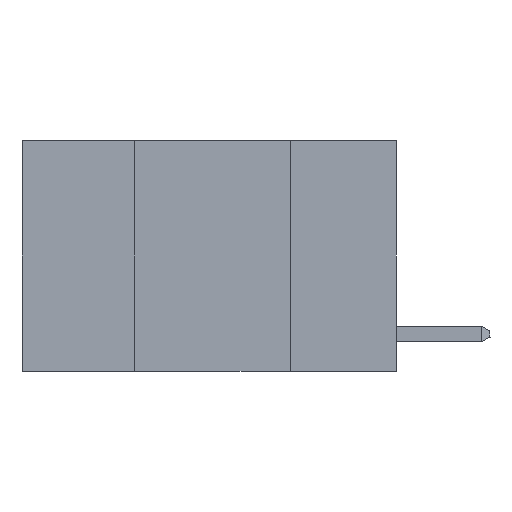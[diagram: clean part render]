
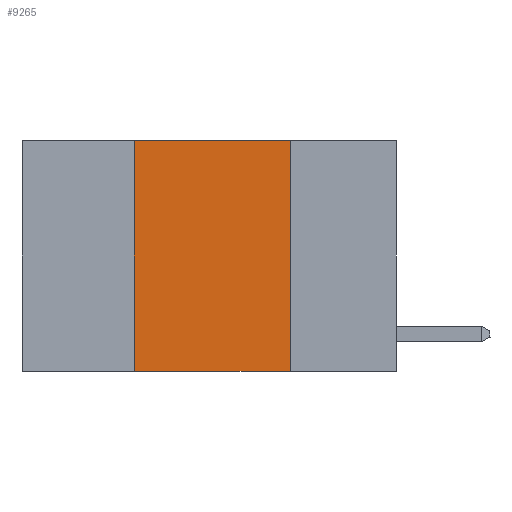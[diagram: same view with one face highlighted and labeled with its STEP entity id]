
A CAD part, left-side view. The second image highlights one B-rep face of the part: STEP entity #9265.
In plain terms, the highlighted planar face has unit normal (-1, 0, 0).
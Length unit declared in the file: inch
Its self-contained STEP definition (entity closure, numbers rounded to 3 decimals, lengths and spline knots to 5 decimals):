
#1022 = EDGE_CURVE ( 'NONE', #4609, #9097, #18171, .T. ) ;
#2296 = ORIENTED_EDGE ( 'NONE', *, *, #17796, .F. ) ;
#2890 = CARTESIAN_POINT ( 'NONE',  ( 0., 0.6, 0. ) ) ;
#3332 = VECTOR ( 'NONE', #21594, 39.37008 ) ;
#4609 = VERTEX_POINT ( 'NONE', #22070 ) ;
#4688 = CARTESIAN_POINT ( 'NONE',  ( 0., 0.42, 0. ) ) ;
#4901 = EDGE_LOOP ( 'NONE', ( #20134, #12432, #2296, #8765 ) ) ;
#5669 = LINE ( 'NONE', #23611, #23332 ) ;
#5858 = DIRECTION ( 'NONE',  ( 0., 0., -1. ) ) ;
#7520 = EDGE_CURVE ( 'NONE', #20606, #9097, #5669, .T. ) ;
#8765 = ORIENTED_EDGE ( 'NONE', *, *, #1022, .T. ) ;
#9097 = VERTEX_POINT ( 'NONE', #20006 ) ;
#9265 = ADVANCED_FACE ( 'NONE', ( #14627 ), #12189, .F. ) ;
#9330 = VECTOR ( 'NONE', #25806, 39.37008 ) ;
#9952 = VECTOR ( 'NONE', #20990, 39.37008 ) ;
#10067 = VERTEX_POINT ( 'NONE', #13952 ) ;
#10439 = DIRECTION ( 'NONE',  ( 1., 0., 0. ) ) ;
#11130 = LINE ( 'NONE', #2890, #9330 ) ;
#11728 = DIRECTION ( 'NONE',  ( 0., 0., -1. ) ) ;
#12189 = PLANE ( 'NONE',  #15612 ) ;
#12432 = ORIENTED_EDGE ( 'NONE', *, *, #18419, .F. ) ;
#13952 = CARTESIAN_POINT ( 'NONE',  ( 0., 0.42, 0. ) ) ;
#14627 = FACE_OUTER_BOUND ( 'NONE', #4901, .T. ) ;
#15612 = AXIS2_PLACEMENT_3D ( 'NONE', #22451, #10439, #5858 ) ;
#17796 = EDGE_CURVE ( 'NONE', #4609, #10067, #22762, .T. ) ;
#18171 = LINE ( 'NONE', #24243, #3332 ) ;
#18419 = EDGE_CURVE ( 'NONE', #10067, #20606, #11130, .T. ) ;
#20006 = CARTESIAN_POINT ( 'NONE',  ( 0., 0.17, -0.37 ) ) ;
#20134 = ORIENTED_EDGE ( 'NONE', *, *, #7520, .F. ) ;
#20606 = VERTEX_POINT ( 'NONE', #25479 ) ;
#20990 = DIRECTION ( 'NONE',  ( 0., 0., 1. ) ) ;
#21594 = DIRECTION ( 'NONE',  ( 0., -1., 0. ) ) ;
#22070 = CARTESIAN_POINT ( 'NONE',  ( 0., 0.42, -0.37 ) ) ;
#22451 = CARTESIAN_POINT ( 'NONE',  ( 0., 0.6, 0. ) ) ;
#22762 = LINE ( 'NONE', #4688, #9952 ) ;
#23332 = VECTOR ( 'NONE', #11728, 39.37008 ) ;
#23611 = CARTESIAN_POINT ( 'NONE',  ( 0., 0.17, 0. ) ) ;
#24243 = CARTESIAN_POINT ( 'NONE',  ( 0., 0.6, -0.37 ) ) ;
#25479 = CARTESIAN_POINT ( 'NONE',  ( 0., 0.17, 0. ) ) ;
#25806 = DIRECTION ( 'NONE',  ( 0., -1., 0. ) ) ;
